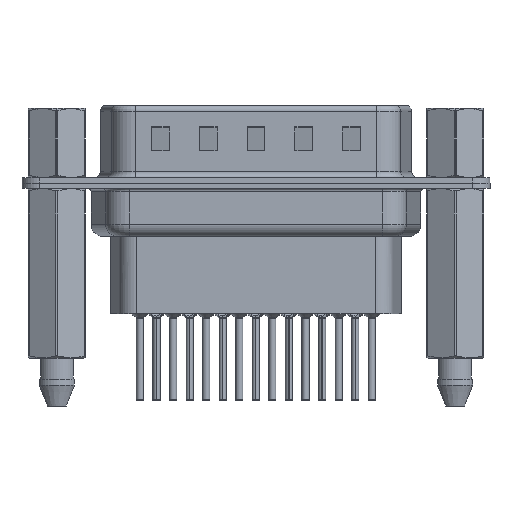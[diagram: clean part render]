
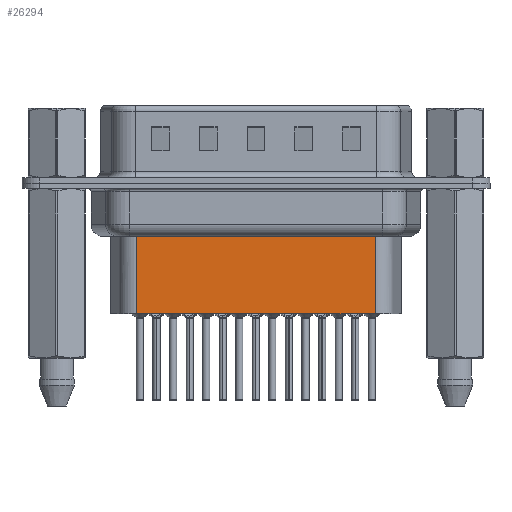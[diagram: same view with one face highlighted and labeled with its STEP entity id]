
A CAD part, front view. The second image highlights one B-rep face of the part: STEP entity #26294.
In plain terms, the highlighted planar face has unit normal (0, -1, 0).
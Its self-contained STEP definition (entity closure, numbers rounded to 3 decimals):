
#1427 = CARTESIAN_POINT ( 'NONE',  ( 26.619, -3.5, -3.1 ) ) ;
#1515 = DIRECTION ( 'NONE',  ( -1., 0., 0. ) ) ;
#2317 = ORIENTED_EDGE ( 'NONE', *, *, #20475, .F. ) ;
#2776 = AXIS2_PLACEMENT_3D ( 'NONE', #23320, #10209, #25525 ) ;
#2907 = VECTOR ( 'NONE', #1515, 1000. ) ;
#5792 = LINE ( 'NONE', #5933, #16177 ) ;
#5933 = CARTESIAN_POINT ( 'NONE',  ( 6.434, -3.5, -4.097 ) ) ;
#7788 = LINE ( 'NONE', #28044, #2907 ) ;
#8172 = ORIENTED_EDGE ( 'NONE', *, *, #11060, .T. ) ;
#9930 = PLANE ( 'NONE',  #2776 ) ;
#10209 = DIRECTION ( 'NONE',  ( 0., -1., 0. ) ) ;
#10730 = DIRECTION ( 'NONE',  ( 0., 0., -1. ) ) ;
#11060 = EDGE_CURVE ( 'NONE', #15922, #20065, #5792, .T. ) ;
#11639 = CARTESIAN_POINT ( 'NONE',  ( 26.619, -3.5, -10.95 ) ) ;
#12061 = ORIENTED_EDGE ( 'NONE', *, *, #16921, .F. ) ;
#12488 = LINE ( 'NONE', #1427, #12796 ) ;
#12796 = VECTOR ( 'NONE', #28101, 1000. ) ;
#13882 = EDGE_LOOP ( 'NONE', ( #2317, #8172, #14172, #12061 ) ) ;
#14145 = FACE_OUTER_BOUND ( 'NONE', #13882, .T. ) ;
#14172 = ORIENTED_EDGE ( 'NONE', *, *, #24850, .T. ) ;
#14940 = DIRECTION ( 'NONE',  ( -1., 0., 0. ) ) ;
#15038 = CARTESIAN_POINT ( 'NONE',  ( 26.619, -3.5, -4.097 ) ) ;
#15515 = LINE ( 'NONE', #17558, #17171 ) ;
#15922 = VERTEX_POINT ( 'NONE', #15038 ) ;
#16177 = VECTOR ( 'NONE', #14940, 1000. ) ;
#16921 = EDGE_CURVE ( 'NONE', #25809, #22703, #7788, .T. ) ;
#17171 = VECTOR ( 'NONE', #10730, 1000. ) ;
#17558 = CARTESIAN_POINT ( 'NONE',  ( 6.681, -3.5, -3.1 ) ) ;
#20065 = VERTEX_POINT ( 'NONE', #22867 ) ;
#20475 = EDGE_CURVE ( 'NONE', #15922, #25809, #12488, .T. ) ;
#22703 = VERTEX_POINT ( 'NONE', #27519 ) ;
#22867 = CARTESIAN_POINT ( 'NONE',  ( 6.681, -3.5, -4.097 ) ) ;
#23320 = CARTESIAN_POINT ( 'NONE',  ( 6.681, -3.5, -3.1 ) ) ;
#24850 = EDGE_CURVE ( 'NONE', #20065, #22703, #15515, .T. ) ;
#25525 = DIRECTION ( 'NONE',  ( 1., 0., 0. ) ) ;
#25809 = VERTEX_POINT ( 'NONE', #11639 ) ;
#26294 = ADVANCED_FACE ( 'NONE', ( #14145 ), #9930, .T. ) ;
#27519 = CARTESIAN_POINT ( 'NONE',  ( 6.681, -3.5, -10.95 ) ) ;
#28044 = CARTESIAN_POINT ( 'NONE',  ( 6.681, -3.5, -10.95 ) ) ;
#28101 = DIRECTION ( 'NONE',  ( 0., 0., -1. ) ) ;
